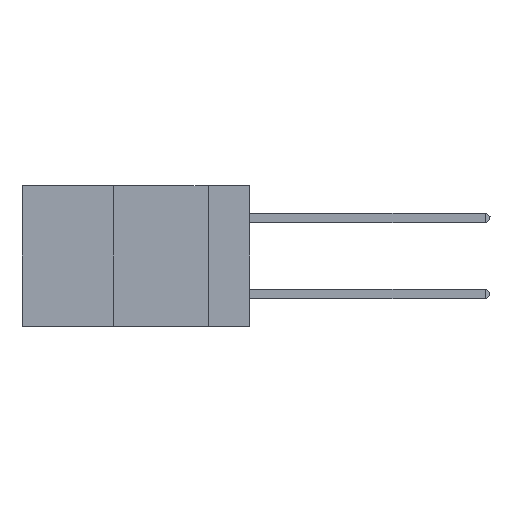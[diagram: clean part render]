
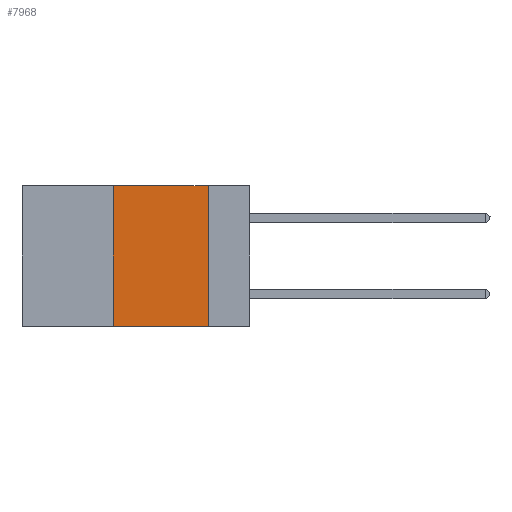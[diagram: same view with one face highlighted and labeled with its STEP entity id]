
A CAD part, left-side view. The second image highlights one B-rep face of the part: STEP entity #7968.
In plain terms, the highlighted planar face has unit normal (-1, 0, 0).
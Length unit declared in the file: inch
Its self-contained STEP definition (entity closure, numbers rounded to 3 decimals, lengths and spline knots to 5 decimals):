
#112 = FACE_OUTER_BOUND ( 'NONE', #8878, .T. ) ;
#323 = VECTOR ( 'NONE', #6611, 39.37008 ) ;
#774 = ORIENTED_EDGE ( 'NONE', *, *, #12853, .F. ) ;
#1710 = DIRECTION ( 'NONE',  ( 0., 0., -1. ) ) ;
#1754 = CARTESIAN_POINT ( 'NONE',  ( 0., 0.6, 0. ) ) ;
#1880 = LINE ( 'NONE', #12514, #323 ) ;
#3352 = EDGE_CURVE ( 'NONE', #8590, #7301, #14716, .T. ) ;
#3685 = VECTOR ( 'NONE', #10147, 39.37008 ) ;
#4137 = LINE ( 'NONE', #5232, #14240 ) ;
#4238 = CARTESIAN_POINT ( 'NONE',  ( 0., 0.11, -0.37 ) ) ;
#5232 = CARTESIAN_POINT ( 'NONE',  ( 0., 0.36, 0. ) ) ;
#5329 = VECTOR ( 'NONE', #1710, 39.37008 ) ;
#5540 = ORIENTED_EDGE ( 'NONE', *, *, #9856, .T. ) ;
#6611 = DIRECTION ( 'NONE',  ( 0., -1., 0. ) ) ;
#7301 = VERTEX_POINT ( 'NONE', #9068 ) ;
#7307 = VERTEX_POINT ( 'NONE', #4238 ) ;
#7398 = DIRECTION ( 'NONE',  ( 1., 0., 0. ) ) ;
#7779 = ORIENTED_EDGE ( 'NONE', *, *, #3352, .F. ) ;
#7968 = ADVANCED_FACE ( 'NONE', ( #112 ), #13318, .F. ) ;
#8590 = VERTEX_POINT ( 'NONE', #14972 ) ;
#8632 = ORIENTED_EDGE ( 'NONE', *, *, #12093, .F. ) ;
#8837 = VERTEX_POINT ( 'NONE', #13178 ) ;
#8878 = EDGE_LOOP ( 'NONE', ( #774, #7779, #8632, #5540 ) ) ;
#9068 = CARTESIAN_POINT ( 'NONE',  ( 0., 0.11, 0. ) ) ;
#9829 = CARTESIAN_POINT ( 'NONE',  ( 0., 0.6, 0. ) ) ;
#9856 = EDGE_CURVE ( 'NONE', #8837, #7307, #1880, .T. ) ;
#10059 = AXIS2_PLACEMENT_3D ( 'NONE', #9829, #7398, #13078 ) ;
#10147 = DIRECTION ( 'NONE',  ( 0., -1., 0. ) ) ;
#10497 = LINE ( 'NONE', #15220, #5329 ) ;
#12093 = EDGE_CURVE ( 'NONE', #8837, #8590, #4137, .T. ) ;
#12514 = CARTESIAN_POINT ( 'NONE',  ( 0., 0.6, -0.37 ) ) ;
#12853 = EDGE_CURVE ( 'NONE', #7301, #7307, #10497, .T. ) ;
#13078 = DIRECTION ( 'NONE',  ( 0., 0., -1. ) ) ;
#13178 = CARTESIAN_POINT ( 'NONE',  ( 0., 0.36, -0.37 ) ) ;
#13318 = PLANE ( 'NONE',  #10059 ) ;
#14240 = VECTOR ( 'NONE', #14707, 39.37008 ) ;
#14707 = DIRECTION ( 'NONE',  ( 0., 0., 1. ) ) ;
#14716 = LINE ( 'NONE', #1754, #3685 ) ;
#14972 = CARTESIAN_POINT ( 'NONE',  ( 0., 0.36, 0. ) ) ;
#15220 = CARTESIAN_POINT ( 'NONE',  ( 0., 0.11, 0. ) ) ;
